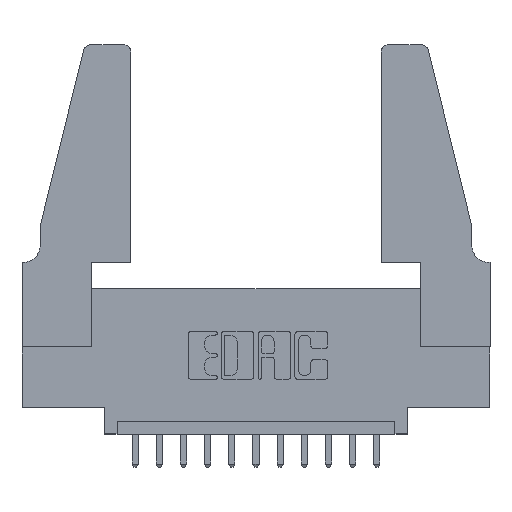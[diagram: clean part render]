
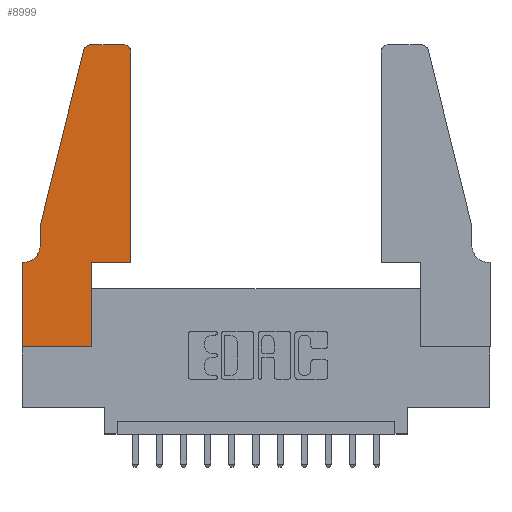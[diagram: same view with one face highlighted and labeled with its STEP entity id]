
A CAD part, top view. The second image highlights one B-rep face of the part: STEP entity #8999.
In plain terms, the highlighted planar face has unit normal (0, 0, 1).
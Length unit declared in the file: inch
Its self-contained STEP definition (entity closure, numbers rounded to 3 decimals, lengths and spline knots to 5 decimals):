
#14 = ORIENTED_EDGE ( 'NONE', *, *, #5780, .T. ) ;
#43 = CARTESIAN_POINT ( 'NONE',  ( 0., 0., 0.37 ) ) ;
#166 = LINE ( 'NONE', #3524, #7365 ) ;
#314 = ORIENTED_EDGE ( 'NONE', *, *, #10161, .T. ) ;
#354 = VECTOR ( 'NONE', #1842, 39.37008 ) ;
#406 = VERTEX_POINT ( 'NONE', #6056 ) ;
#461 = CARTESIAN_POINT ( 'NONE',  ( 0.2605, 1.25, 0.37 ) ) ;
#861 = CARTESIAN_POINT ( 'NONE',  ( 0.2865, 0.35, 0.37 ) ) ;
#1087 = LINE ( 'NONE', #461, #10209 ) ;
#1360 = LINE ( 'NONE', #11167, #4804 ) ;
#1745 = VERTEX_POINT ( 'NONE', #3932 ) ;
#1842 = DIRECTION ( 'NONE',  ( 1., 0., 0. ) ) ;
#1962 = DIRECTION ( 'NONE',  ( -1., 0., 0. ) ) ;
#2218 = CARTESIAN_POINT ( 'NONE',  ( 0.284, 1.25, 0.37 ) ) ;
#2460 = EDGE_CURVE ( 'NONE', #406, #4526, #2690, .T. ) ;
#2525 = CARTESIAN_POINT ( 'NONE',  ( 0.4505, 1.22, 0.37 ) ) ;
#2683 = CIRCLE ( 'NONE', #11967, 0.03 ) ;
#2690 = CIRCLE ( 'NONE', #2754, 0.07 ) ;
#2747 = EDGE_CURVE ( 'NONE', #3550, #406, #14614, .T. ) ;
#2754 = AXIS2_PLACEMENT_3D ( 'NONE', #4159, #9957, #2912 ) ;
#2825 = CARTESIAN_POINT ( 'NONE',  ( 0., 0., 0.37 ) ) ;
#2912 = DIRECTION ( 'NONE',  ( -1., 0., 0. ) ) ;
#2943 = VECTOR ( 'NONE', #9666, 39.37008 ) ;
#3199 = EDGE_CURVE ( 'NONE', #4311, #6006, #8034, .T. ) ;
#3454 = ORIENTED_EDGE ( 'NONE', *, *, #3199, .T. ) ;
#3524 = CARTESIAN_POINT ( 'NONE',  ( 0., 0., 0.37 ) ) ;
#3550 = VERTEX_POINT ( 'NONE', #7933 ) ;
#3765 = CARTESIAN_POINT ( 'NONE',  ( 0.4505, 0.35, 0.37 ) ) ;
#3932 = CARTESIAN_POINT ( 'NONE',  ( 0.25487, 1.22718, 0.37 ) ) ;
#3970 = VERTEX_POINT ( 'NONE', #8848 ) ;
#4052 = DIRECTION ( 'NONE',  ( -1., 0., 0. ) ) ;
#4159 = CARTESIAN_POINT ( 'NONE',  ( 0.0055, 0.42, 0.37 ) ) ;
#4311 = VERTEX_POINT ( 'NONE', #6580 ) ;
#4331 = EDGE_CURVE ( 'NONE', #4526, #3970, #1360, .T. ) ;
#4509 = LINE ( 'NONE', #9888, #354 ) ;
#4526 = VERTEX_POINT ( 'NONE', #10119 ) ;
#4667 = EDGE_CURVE ( 'NONE', #7917, #10341, #7468, .T. ) ;
#4725 = DIRECTION ( 'NONE',  ( 1., 0., 0. ) ) ;
#4804 = VECTOR ( 'NONE', #1962, 39.37008 ) ;
#4834 = ORIENTED_EDGE ( 'NONE', *, *, #12750, .T. ) ;
#4938 = DIRECTION ( 'NONE',  ( 0., -1., 0. ) ) ;
#5058 = DIRECTION ( 'NONE',  ( 0., 0., 1. ) ) ;
#5158 = DIRECTION ( 'NONE',  ( 1., 0., 0. ) ) ;
#5643 = AXIS2_PLACEMENT_3D ( 'NONE', #7356, #14168, #5158 ) ;
#5734 = CARTESIAN_POINT ( 'NONE',  ( 0.2865, 0.35, 0.37 ) ) ;
#5754 = FACE_OUTER_BOUND ( 'NONE', #13842, .T. ) ;
#5780 = EDGE_CURVE ( 'NONE', #1745, #3550, #6373, .T. ) ;
#5813 = VERTEX_POINT ( 'NONE', #2825 ) ;
#6006 = VERTEX_POINT ( 'NONE', #861 ) ;
#6056 = CARTESIAN_POINT ( 'NONE',  ( 0.0755, 0.42, 0.37 ) ) ;
#6189 = ORIENTED_EDGE ( 'NONE', *, *, #2460, .T. ) ;
#6203 = PLANE ( 'NONE',  #5643 ) ;
#6373 = LINE ( 'NONE', #10844, #2943 ) ;
#6395 = VERTEX_POINT ( 'NONE', #3765 ) ;
#6431 = ORIENTED_EDGE ( 'NONE', *, *, #11411, .T. ) ;
#6580 = CARTESIAN_POINT ( 'NONE',  ( 0.2865, 0., 0.37 ) ) ;
#6618 = ORIENTED_EDGE ( 'NONE', *, *, #4331, .T. ) ;
#7022 = ORIENTED_EDGE ( 'NONE', *, *, #2747, .T. ) ;
#7356 = CARTESIAN_POINT ( 'NONE',  ( 0., 0.35, 0.37 ) ) ;
#7365 = VECTOR ( 'NONE', #4725, 39.37008 ) ;
#7468 = CIRCLE ( 'NONE', #14015, 0.03 ) ;
#7594 = CARTESIAN_POINT ( 'NONE',  ( 0.4505, 0.35, 0.37 ) ) ;
#7858 = VECTOR ( 'NONE', #12500, 39.37008 ) ;
#7917 = VERTEX_POINT ( 'NONE', #2525 ) ;
#7933 = CARTESIAN_POINT ( 'NONE',  ( 0.0755, 0.5, 0.37 ) ) ;
#8034 = LINE ( 'NONE', #5734, #7858 ) ;
#8480 = CARTESIAN_POINT ( 'NONE',  ( 0.0755, 0.5, 0.37 ) ) ;
#8522 = VERTEX_POINT ( 'NONE', #2218 ) ;
#8574 = DIRECTION ( 'NONE',  ( 0., -1., 0. ) ) ;
#8667 = EDGE_CURVE ( 'NONE', #5813, #4311, #166, .T. ) ;
#8698 = CARTESIAN_POINT ( 'NONE',  ( 0.284, 1.22, 0.37 ) ) ;
#8806 = DIRECTION ( 'NONE',  ( 0., 1., 0. ) ) ;
#8848 = CARTESIAN_POINT ( 'NONE',  ( 0., 0.35, 0.37 ) ) ;
#8940 = ORIENTED_EDGE ( 'NONE', *, *, #4667, .T. ) ;
#8999 = ADVANCED_FACE ( 'NONE', ( #5754 ), #6203, .T. ) ;
#9060 = EDGE_CURVE ( 'NONE', #8522, #1745, #2683, .T. ) ;
#9095 = ORIENTED_EDGE ( 'NONE', *, *, #9060, .T. ) ;
#9666 = DIRECTION ( 'NONE',  ( -0.239, -0.971, 0. ) ) ;
#9811 = VECTOR ( 'NONE', #8574, 39.37008 ) ;
#9842 = DIRECTION ( 'NONE',  ( 1., 0., 0. ) ) ;
#9888 = CARTESIAN_POINT ( 'NONE',  ( 0.4505, 0.35, 0.37 ) ) ;
#9957 = DIRECTION ( 'NONE',  ( 0., 0., -1. ) ) ;
#10119 = CARTESIAN_POINT ( 'NONE',  ( 0.0055, 0.35, 0.37 ) ) ;
#10161 = EDGE_CURVE ( 'NONE', #6395, #7917, #14018, .T. ) ;
#10209 = VECTOR ( 'NONE', #4052, 39.37008 ) ;
#10341 = VERTEX_POINT ( 'NONE', #12397 ) ;
#10844 = CARTESIAN_POINT ( 'NONE',  ( 0.0755, 0.5, 0.37 ) ) ;
#10927 = DIRECTION ( 'NONE',  ( 0., 0., 1. ) ) ;
#11167 = CARTESIAN_POINT ( 'NONE',  ( 0.0755, 0.35, 0.37 ) ) ;
#11411 = EDGE_CURVE ( 'NONE', #10341, #8522, #1087, .T. ) ;
#11967 = AXIS2_PLACEMENT_3D ( 'NONE', #8698, #5058, #12960 ) ;
#12262 = EDGE_CURVE ( 'NONE', #6006, #6395, #4509, .T. ) ;
#12295 = LINE ( 'NONE', #43, #12991 ) ;
#12397 = CARTESIAN_POINT ( 'NONE',  ( 0.4205, 1.25, 0.37 ) ) ;
#12500 = DIRECTION ( 'NONE',  ( 0., 1., 0. ) ) ;
#12750 = EDGE_CURVE ( 'NONE', #3970, #5813, #12295, .T. ) ;
#12960 = DIRECTION ( 'NONE',  ( 1., 0., 0. ) ) ;
#12991 = VECTOR ( 'NONE', #4938, 39.37008 ) ;
#13014 = ORIENTED_EDGE ( 'NONE', *, *, #12262, .T. ) ;
#13040 = CARTESIAN_POINT ( 'NONE',  ( 0.4205, 1.22, 0.37 ) ) ;
#13771 = ORIENTED_EDGE ( 'NONE', *, *, #8667, .T. ) ;
#13842 = EDGE_LOOP ( 'NONE', ( #6431, #9095, #14, #7022, #6189, #6618, #4834, #13771, #3454, #13014, #314, #8940 ) ) ;
#14015 = AXIS2_PLACEMENT_3D ( 'NONE', #13040, #10927, #9842 ) ;
#14018 = LINE ( 'NONE', #7594, #14388 ) ;
#14168 = DIRECTION ( 'NONE',  ( 0., 0., 1. ) ) ;
#14388 = VECTOR ( 'NONE', #8806, 39.37008 ) ;
#14614 = LINE ( 'NONE', #8480, #9811 ) ;
